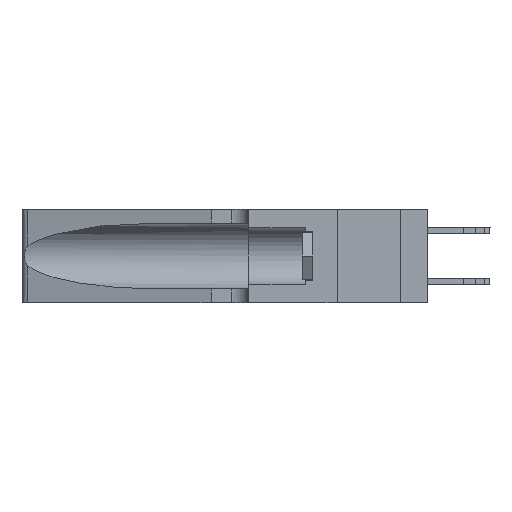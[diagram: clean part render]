
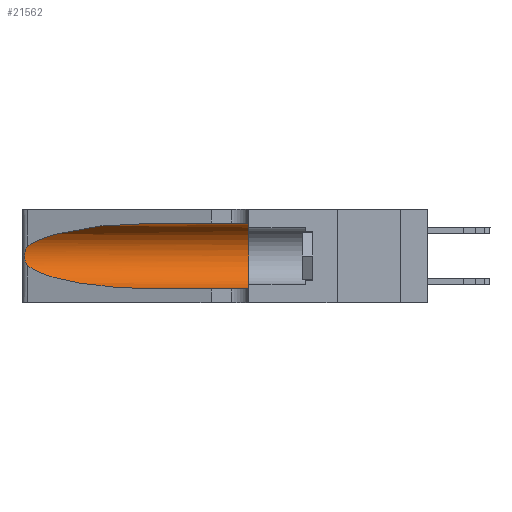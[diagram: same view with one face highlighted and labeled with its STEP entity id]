
A CAD part, left-side view. The second image highlights one B-rep face of the part: STEP entity #21562.
In plain terms, the highlighted cylindrical face has radius 3.308 mm (diameter 6.617 mm), a partial arc.
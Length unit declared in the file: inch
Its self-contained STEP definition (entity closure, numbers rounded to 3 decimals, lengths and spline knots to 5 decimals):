
#296 = VERTEX_POINT ( 'NONE', #31976 ) ;
#362 = EDGE_LOOP ( 'NONE', ( #21782, #22113, #5691, #17477, #28301, #11018 ) ) ;
#1696 = DIRECTION ( 'NONE',  ( 0., -1., 0. ) ) ;
#3215 = CARTESIAN_POINT ( 'NONE',  ( 0.25555, 1.22993, 0.14849 ) ) ;
#3982 = CARTESIAN_POINT ( 'NONE',  ( 0.2373, 1.15595, 0.28018 ) ) ;
#5691 = ORIENTED_EDGE ( 'NONE', *, *, #16089, .T. ) ;
#6084 = CARTESIAN_POINT ( 'NONE',  ( 0.1305, 1.61858, 0.185 ) ) ;
#8003 = EDGE_CURVE ( 'NONE', #27901, #22369, #14930, .T. ) ;
#8416 = CIRCLE ( 'NONE', #11907, 0.13025 ) ;
#8678 = VECTOR ( 'NONE', #26512, 39.37008 ) ;
#8694 = CARTESIAN_POINT ( 'NONE',  ( 0.25856, 1.23593, 0.16098 ) ) ;
#9297 = AXIS2_PLACEMENT_3D ( 'NONE', #6084, #37109, #31648 ) ;
#9523 = CARTESIAN_POINT ( 'NONE',  ( 0.25487, 1.22718, 0.14631 ) ) ;
#9781 = CARTESIAN_POINT ( 'NONE',  ( 0.1305, 1.61858, 0.31525 ) ) ;
#10001 = CARTESIAN_POINT ( 'NONE',  ( 0.25487, 1.22718, 0.22369 ) ) ;
#10623 = FACE_OUTER_BOUND ( 'NONE', #362, .T. ) ;
#11018 = ORIENTED_EDGE ( 'NONE', *, *, #34417, .F. ) ;
#11732 = CARTESIAN_POINT ( 'NONE',  ( 0.1305, 0.72297, 0.31525 ) ) ;
#11907 = AXIS2_PLACEMENT_3D ( 'NONE', #16594, #33839, #19455 ) ;
#11936 = CYLINDRICAL_SURFACE ( 'NONE', #9297, 0.13025 ) ;
#12394 = CARTESIAN_POINT ( 'NONE',  ( 0.18966, 0.96281, 0.05475 ) ) ;
#14930 = B_SPLINE_CURVE_WITH_KNOTS ( 'NONE', 3,
 ( #25013, #25333, #19218, #25215, #30772, #16587, #17172, #31409, #34234, #8694, #28591, #20208, #3215, #32262 ),
 .UNSPECIFIED., .F., .F.,
 ( 4, 2, 2, 2, 2, 2, 4 ),
 ( 0., 0.00027, 0.00053, 0.00107, 0.0016, 0.00187, 0.00214 ),
 .UNSPECIFIED. ) ;
#15600 = EDGE_CURVE ( 'NONE', #296, #27901, #26404, .T. ) ;
#16089 = EDGE_CURVE ( 'NONE', #22369, #23323, #20896, .T. ) ;
#16587 = CARTESIAN_POINT ( 'NONE',  ( 0.26018, 1.23835, 0.19895 ) ) ;
#16594 = CARTESIAN_POINT ( 'NONE',  ( 0.1305, 0.35, 0.185 ) ) ;
#16973 = EDGE_CURVE ( 'NONE', #23323, #35459, #21065, .T. ) ;
#17172 = CARTESIAN_POINT ( 'NONE',  ( 0.26075, 1.23896, 0.19203 ) ) ;
#17477 = ORIENTED_EDGE ( 'NONE', *, *, #16973, .T. ) ;
#17900 = CARTESIAN_POINT ( 'NONE',  ( 0.1305, 0.35, 0.31525 ) ) ;
#18111 = CARTESIAN_POINT ( 'NONE',  ( 0.1305, 0.72297, 0.05475 ) ) ;
#18643 = CARTESIAN_POINT ( 'NONE',  ( 0.1305, 1.61858, 0.05475 ) ) ;
#19218 = CARTESIAN_POINT ( 'NONE',  ( 0.25639, 1.23184, 0.21858 ) ) ;
#19455 = DIRECTION ( 'NONE',  ( 0., 0., 1. ) ) ;
#20208 = CARTESIAN_POINT ( 'NONE',  ( 0.25639, 1.23186, 0.15144 ) ) ;
#20896 =( BOUNDED_CURVE ( )  B_SPLINE_CURVE ( 3, ( #9523, #29679, #12394, #18111 ),
 .UNSPECIFIED., .F., .F. ) 
 B_SPLINE_CURVE_WITH_KNOTS ( ( 4, 4 ),
 ( 3.44316, 4.71239 ),
 .UNSPECIFIED. ) 
 CURVE ( )  GEOMETRIC_REPRESENTATION_ITEM ( )  RATIONAL_B_SPLINE_CURVE ( ( 1., 0.87, 0.87, 1. ) ) 
 REPRESENTATION_ITEM ( '' )  );
#21065 = LINE ( 'NONE', #18643, #22420 ) ;
#21339 = EDGE_CURVE ( 'NONE', #24782, #35459, #8416, .T. ) ;
#21562 = ADVANCED_FACE ( 'NONE', ( #10623 ), #11936, .F. ) ;
#21594 = CARTESIAN_POINT ( 'NONE',  ( 0.1305, 0.72297, 0.05475 ) ) ;
#21782 = ORIENTED_EDGE ( 'NONE', *, *, #15600, .T. ) ;
#22113 = ORIENTED_EDGE ( 'NONE', *, *, #8003, .T. ) ;
#22369 = VERTEX_POINT ( 'NONE', #23516 ) ;
#22420 = VECTOR ( 'NONE', #1696, 39.37008 ) ;
#23323 = VERTEX_POINT ( 'NONE', #21594 ) ;
#23516 = CARTESIAN_POINT ( 'NONE',  ( 0.25487, 1.22718, 0.14631 ) ) ;
#24782 = VERTEX_POINT ( 'NONE', #17900 ) ;
#25013 = CARTESIAN_POINT ( 'NONE',  ( 0.25487, 1.22718, 0.22369 ) ) ;
#25215 = CARTESIAN_POINT ( 'NONE',  ( 0.25787, 1.23484, 0.2124 ) ) ;
#25333 = CARTESIAN_POINT ( 'NONE',  ( 0.25555, 1.22994, 0.2215 ) ) ;
#25687 = LINE ( 'NONE', #9781, #8678 ) ;
#26404 =( BOUNDED_CURVE ( )  B_SPLINE_CURVE ( 3, ( #11732, #26963, #3982, #29233 ),
 .UNSPECIFIED., .F., .T. ) 
 B_SPLINE_CURVE_WITH_KNOTS ( ( 4, 4 ),
 ( 1.5708, 2.84003 ),
 .UNSPECIFIED. ) 
 CURVE ( )  GEOMETRIC_REPRESENTATION_ITEM ( )  RATIONAL_B_SPLINE_CURVE ( ( 1., 0.87, 0.87, 1. ) ) 
 REPRESENTATION_ITEM ( '' )  );
#26512 = DIRECTION ( 'NONE',  ( 0., -1., 0. ) ) ;
#26963 = CARTESIAN_POINT ( 'NONE',  ( 0.18966, 0.96281, 0.31525 ) ) ;
#27901 = VERTEX_POINT ( 'NONE', #10001 ) ;
#28261 = CARTESIAN_POINT ( 'NONE',  ( 0.1305, 0.35, 0.05475 ) ) ;
#28301 = ORIENTED_EDGE ( 'NONE', *, *, #21339, .F. ) ;
#28591 = CARTESIAN_POINT ( 'NONE',  ( 0.25789, 1.23486, 0.15765 ) ) ;
#29233 = CARTESIAN_POINT ( 'NONE',  ( 0.25487, 1.22718, 0.22369 ) ) ;
#29679 = CARTESIAN_POINT ( 'NONE',  ( 0.2373, 1.15595, 0.08982 ) ) ;
#30772 = CARTESIAN_POINT ( 'NONE',  ( 0.25854, 1.2359, 0.20912 ) ) ;
#31409 = CARTESIAN_POINT ( 'NONE',  ( 0.26075, 1.23896, 0.178 ) ) ;
#31648 = DIRECTION ( 'NONE',  ( 0., 0., -1. ) ) ;
#31976 = CARTESIAN_POINT ( 'NONE',  ( 0.1305, 0.72297, 0.31525 ) ) ;
#32262 = CARTESIAN_POINT ( 'NONE',  ( 0.25487, 1.22718, 0.14631 ) ) ;
#33839 = DIRECTION ( 'NONE',  ( 0., 1., 0. ) ) ;
#34234 = CARTESIAN_POINT ( 'NONE',  ( 0.26017, 1.23833, 0.17102 ) ) ;
#34417 = EDGE_CURVE ( 'NONE', #296, #24782, #25687, .T. ) ;
#35459 = VERTEX_POINT ( 'NONE', #28261 ) ;
#37109 = DIRECTION ( 'NONE',  ( 0., -1., 0. ) ) ;
